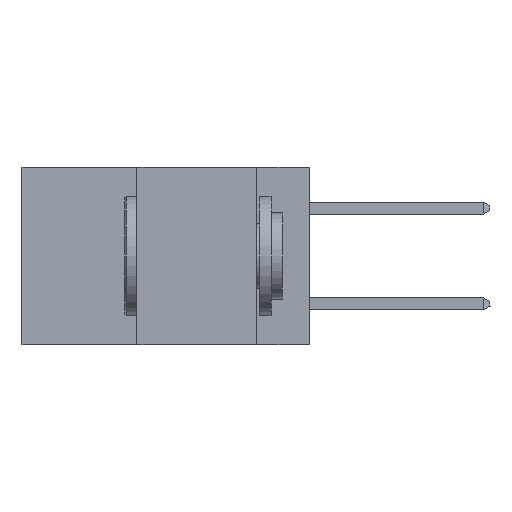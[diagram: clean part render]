
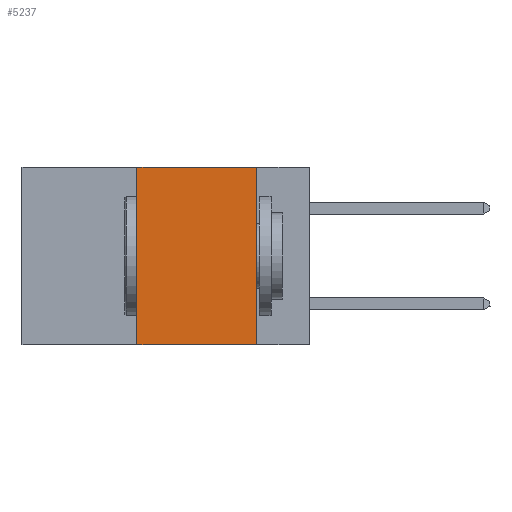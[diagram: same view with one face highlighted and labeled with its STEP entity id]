
A CAD part, left-side view. The second image highlights one B-rep face of the part: STEP entity #5237.
In plain terms, the highlighted planar face has unit normal (-1, 0, 0).
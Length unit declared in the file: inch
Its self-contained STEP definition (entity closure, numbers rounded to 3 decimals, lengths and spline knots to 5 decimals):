
#1090 = VECTOR ( 'NONE', #2867, 39.37008 ) ;
#2867 = DIRECTION ( 'NONE',  ( 0., 0., 1. ) ) ;
#3658 = CARTESIAN_POINT ( 'NONE',  ( 0., 0.6, 0. ) ) ;
#5209 = CARTESIAN_POINT ( 'NONE',  ( 0., 0.36, -0.37 ) ) ;
#5237 = ADVANCED_FACE ( 'NONE', ( #15920 ), #18183, .F. ) ;
#6694 = ORIENTED_EDGE ( 'NONE', *, *, #24539, .F. ) ;
#6804 = CARTESIAN_POINT ( 'NONE',  ( 0., 0.36, 0. ) ) ;
#6958 = ORIENTED_EDGE ( 'NONE', *, *, #31026, .T. ) ;
#7470 = DIRECTION ( 'NONE',  ( 1., 0., 0. ) ) ;
#8758 = ORIENTED_EDGE ( 'NONE', *, *, #17233, .F. ) ;
#9409 = CARTESIAN_POINT ( 'NONE',  ( 0., 0.11, 0. ) ) ;
#9942 = AXIS2_PLACEMENT_3D ( 'NONE', #14777, #7470, #30212 ) ;
#10125 = DIRECTION ( 'NONE',  ( 0., 0., -1. ) ) ;
#11797 = CARTESIAN_POINT ( 'NONE',  ( 0., 0.11, 0. ) ) ;
#12611 = VERTEX_POINT ( 'NONE', #6804 ) ;
#14286 = ORIENTED_EDGE ( 'NONE', *, *, #17447, .F. ) ;
#14334 = CARTESIAN_POINT ( 'NONE',  ( 0., 0.6, -0.37 ) ) ;
#14777 = CARTESIAN_POINT ( 'NONE',  ( 0., 0.6, 0. ) ) ;
#15316 = CARTESIAN_POINT ( 'NONE',  ( 0., 0.36, 0. ) ) ;
#15920 = FACE_OUTER_BOUND ( 'NONE', #26300, .T. ) ;
#17233 = EDGE_CURVE ( 'NONE', #25265, #12611, #27254, .T. ) ;
#17447 = EDGE_CURVE ( 'NONE', #12611, #20057, #28809, .T. ) ;
#18183 = PLANE ( 'NONE',  #9942 ) ;
#19960 = DIRECTION ( 'NONE',  ( 0., -1., 0. ) ) ;
#20057 = VERTEX_POINT ( 'NONE', #11797 ) ;
#21118 = VERTEX_POINT ( 'NONE', #22995 ) ;
#22235 = VECTOR ( 'NONE', #26371, 39.37008 ) ;
#22995 = CARTESIAN_POINT ( 'NONE',  ( 0., 0.11, -0.37 ) ) ;
#24539 = EDGE_CURVE ( 'NONE', #20057, #21118, #31352, .T. ) ;
#25265 = VERTEX_POINT ( 'NONE', #5209 ) ;
#26300 = EDGE_LOOP ( 'NONE', ( #6694, #14286, #8758, #6958 ) ) ;
#26371 = DIRECTION ( 'NONE',  ( 0., -1., 0. ) ) ;
#27254 = LINE ( 'NONE', #15316, #1090 ) ;
#28778 = LINE ( 'NONE', #14334, #22235 ) ;
#28809 = LINE ( 'NONE', #3658, #30665 ) ;
#30158 = VECTOR ( 'NONE', #10125, 39.37008 ) ;
#30212 = DIRECTION ( 'NONE',  ( 0., 0., -1. ) ) ;
#30665 = VECTOR ( 'NONE', #19960, 39.37008 ) ;
#31026 = EDGE_CURVE ( 'NONE', #25265, #21118, #28778, .T. ) ;
#31352 = LINE ( 'NONE', #9409, #30158 ) ;
